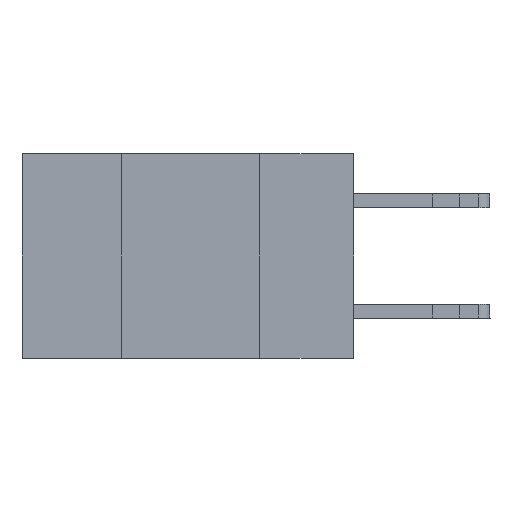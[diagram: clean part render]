
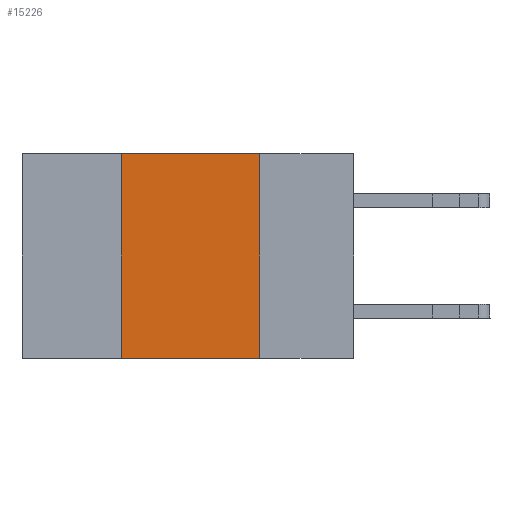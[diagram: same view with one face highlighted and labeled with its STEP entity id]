
A CAD part, left-side view. The second image highlights one B-rep face of the part: STEP entity #15226.
In plain terms, the highlighted planar face has unit normal (-1, 0, 0).
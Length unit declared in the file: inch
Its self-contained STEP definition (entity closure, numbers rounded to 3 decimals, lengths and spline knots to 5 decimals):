
#245 = DIRECTION ( 'NONE',  ( 1., 0., 0. ) ) ;
#728 = VECTOR ( 'NONE', #9614, 39.37008 ) ;
#1270 = CARTESIAN_POINT ( 'NONE',  ( 0., 0.42, -0.37 ) ) ;
#1759 = VERTEX_POINT ( 'NONE', #7605 ) ;
#2521 = CARTESIAN_POINT ( 'NONE',  ( 0., 0.42, 0. ) ) ;
#2576 = EDGE_LOOP ( 'NONE', ( #5698, #16117, #16549, #6562 ) ) ;
#2642 = DIRECTION ( 'NONE',  ( 0., -1., 0. ) ) ;
#3667 = EDGE_CURVE ( 'NONE', #16385, #1759, #8976, .T. ) ;
#4393 = VERTEX_POINT ( 'NONE', #17234 ) ;
#4656 = EDGE_CURVE ( 'NONE', #16385, #6855, #11120, .T. ) ;
#5555 = EDGE_CURVE ( 'NONE', #4393, #6855, #13846, .T. ) ;
#5698 = ORIENTED_EDGE ( 'NONE', *, *, #5555, .F. ) ;
#6562 = ORIENTED_EDGE ( 'NONE', *, *, #4656, .T. ) ;
#6855 = VERTEX_POINT ( 'NONE', #16817 ) ;
#7605 = CARTESIAN_POINT ( 'NONE',  ( 0., 0.42, 0. ) ) ;
#7651 = EDGE_CURVE ( 'NONE', #1759, #4393, #15817, .T. ) ;
#8300 = AXIS2_PLACEMENT_3D ( 'NONE', #14955, #245, #9858 ) ;
#8545 = PLANE ( 'NONE',  #8300 ) ;
#8976 = LINE ( 'NONE', #2521, #14995 ) ;
#9614 = DIRECTION ( 'NONE',  ( 0., -1., 0. ) ) ;
#9649 = CARTESIAN_POINT ( 'NONE',  ( 0., 0.6, -0.37 ) ) ;
#9858 = DIRECTION ( 'NONE',  ( 0., 0., -1. ) ) ;
#11120 = LINE ( 'NONE', #9649, #728 ) ;
#12010 = CARTESIAN_POINT ( 'NONE',  ( 0., 0.6, 0. ) ) ;
#12348 = VECTOR ( 'NONE', #2642, 39.37008 ) ;
#12901 = CARTESIAN_POINT ( 'NONE',  ( 0., 0.17, 0. ) ) ;
#13846 = LINE ( 'NONE', #12901, #16968 ) ;
#14955 = CARTESIAN_POINT ( 'NONE',  ( 0., 0.6, 0. ) ) ;
#14995 = VECTOR ( 'NONE', #16103, 39.37008 ) ;
#15148 = FACE_OUTER_BOUND ( 'NONE', #2576, .T. ) ;
#15226 = ADVANCED_FACE ( 'NONE', ( #15148 ), #8545, .F. ) ;
#15530 = DIRECTION ( 'NONE',  ( 0., 0., -1. ) ) ;
#15817 = LINE ( 'NONE', #12010, #12348 ) ;
#16103 = DIRECTION ( 'NONE',  ( 0., 0., 1. ) ) ;
#16117 = ORIENTED_EDGE ( 'NONE', *, *, #7651, .F. ) ;
#16385 = VERTEX_POINT ( 'NONE', #1270 ) ;
#16549 = ORIENTED_EDGE ( 'NONE', *, *, #3667, .F. ) ;
#16817 = CARTESIAN_POINT ( 'NONE',  ( 0., 0.17, -0.37 ) ) ;
#16968 = VECTOR ( 'NONE', #15530, 39.37008 ) ;
#17234 = CARTESIAN_POINT ( 'NONE',  ( 0., 0.17, 0. ) ) ;
